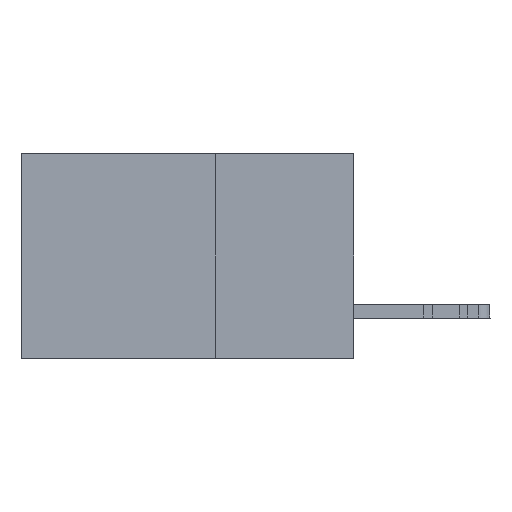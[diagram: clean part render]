
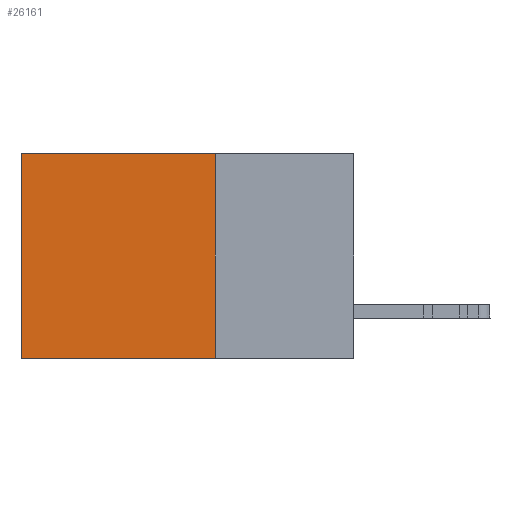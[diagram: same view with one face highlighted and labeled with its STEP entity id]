
A CAD part, left-side view. The second image highlights one B-rep face of the part: STEP entity #26161.
In plain terms, the highlighted planar face has unit normal (-1, 0, 0).
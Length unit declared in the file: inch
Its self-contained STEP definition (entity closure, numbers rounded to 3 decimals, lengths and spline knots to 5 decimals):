
#192 = VERTEX_POINT ( 'NONE', #14217 ) ;
#1455 = DIRECTION ( 'NONE',  ( 1., 0., 0. ) ) ;
#5048 = DIRECTION ( 'NONE',  ( 0., 0., -1. ) ) ;
#5794 = DIRECTION ( 'NONE',  ( 0., 1., 0. ) ) ;
#10250 = VERTEX_POINT ( 'NONE', #25502 ) ;
#10639 = LINE ( 'NONE', #18542, #47404 ) ;
#13328 = CARTESIAN_POINT ( 'NONE',  ( 0.2875, 0.25, 0. ) ) ;
#13860 = CARTESIAN_POINT ( 'NONE',  ( 0.2875, 0.25, -0.37 ) ) ;
#13987 = CARTESIAN_POINT ( 'NONE',  ( 0.2875, 0.25, -0.37 ) ) ;
#14217 = CARTESIAN_POINT ( 'NONE',  ( 0.2875, 0.6, -0.37 ) ) ;
#16519 = VERTEX_POINT ( 'NONE', #13328 ) ;
#18542 = CARTESIAN_POINT ( 'NONE',  ( 0.2875, 0.25, 0. ) ) ;
#19663 = FACE_OUTER_BOUND ( 'NONE', #47203, .T. ) ;
#23142 = EDGE_CURVE ( 'NONE', #10250, #192, #36425, .T. ) ;
#25502 = CARTESIAN_POINT ( 'NONE',  ( 0.2875, 0.6, 0. ) ) ;
#26161 = ADVANCED_FACE ( 'NONE', ( #19663 ), #34305, .F. ) ;
#27588 = VERTEX_POINT ( 'NONE', #13860 ) ;
#28148 = DIRECTION ( 'NONE',  ( 0., 1., 0. ) ) ;
#28477 = VECTOR ( 'NONE', #29205, 39.37008 ) ;
#28646 = EDGE_CURVE ( 'NONE', #16519, #27588, #10639, .T. ) ;
#29205 = DIRECTION ( 'NONE',  ( 0., 0., -1. ) ) ;
#31987 = LINE ( 'NONE', #13987, #32441 ) ;
#32441 = VECTOR ( 'NONE', #28148, 39.37008 ) ;
#34071 = CARTESIAN_POINT ( 'NONE',  ( 0.2875, 0.25, 0. ) ) ;
#34305 = PLANE ( 'NONE',  #44058 ) ;
#35294 = ORIENTED_EDGE ( 'NONE', *, *, #23142, .T. ) ;
#36416 = EDGE_CURVE ( 'NONE', #27588, #192, #31987, .T. ) ;
#36425 = LINE ( 'NONE', #40022, #28477 ) ;
#36521 = ORIENTED_EDGE ( 'NONE', *, *, #36416, .F. ) ;
#38494 = ORIENTED_EDGE ( 'NONE', *, *, #44472, .T. ) ;
#38681 = LINE ( 'NONE', #45654, #40254 ) ;
#40022 = CARTESIAN_POINT ( 'NONE',  ( 0.2875, 0.6, 0. ) ) ;
#40254 = VECTOR ( 'NONE', #5794, 39.37008 ) ;
#43278 = DIRECTION ( 'NONE',  ( 0., 0., -1. ) ) ;
#44058 = AXIS2_PLACEMENT_3D ( 'NONE', #34071, #1455, #5048 ) ;
#44472 = EDGE_CURVE ( 'NONE', #16519, #10250, #38681, .T. ) ;
#45654 = CARTESIAN_POINT ( 'NONE',  ( 0.2875, 0.25, 0. ) ) ;
#46265 = ORIENTED_EDGE ( 'NONE', *, *, #28646, .F. ) ;
#47203 = EDGE_LOOP ( 'NONE', ( #35294, #36521, #46265, #38494 ) ) ;
#47404 = VECTOR ( 'NONE', #43278, 39.37008 ) ;
